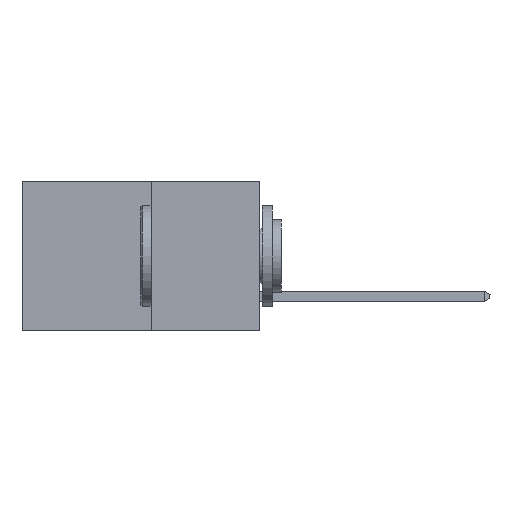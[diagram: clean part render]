
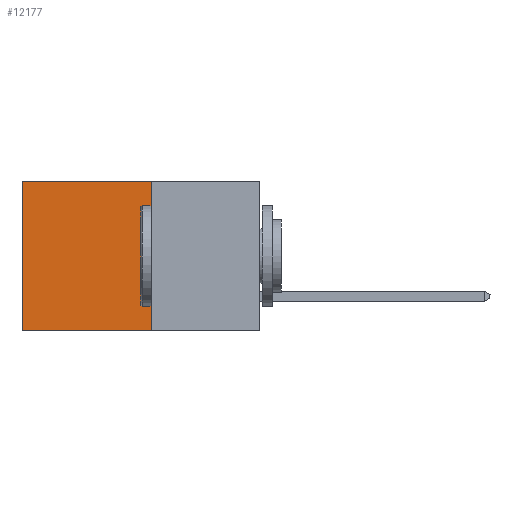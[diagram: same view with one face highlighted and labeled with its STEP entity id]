
A CAD part, left-side view. The second image highlights one B-rep face of the part: STEP entity #12177.
In plain terms, the highlighted planar face has unit normal (-1, 0, 0).
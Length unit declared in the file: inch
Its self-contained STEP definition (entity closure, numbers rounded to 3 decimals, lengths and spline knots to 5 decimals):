
#56 = LINE ( 'NONE', #4980, #15350 ) ;
#173 = VERTEX_POINT ( 'NONE', #7749 ) ;
#834 = ORIENTED_EDGE ( 'NONE', *, *, #2301, .F. ) ;
#1101 = PLANE ( 'NONE',  #8756 ) ;
#1112 = DIRECTION ( 'NONE',  ( 0., 0., -1. ) ) ;
#1713 = LINE ( 'NONE', #13297, #14385 ) ;
#1985 = EDGE_LOOP ( 'NONE', ( #5039, #834, #10351, #9979 ) ) ;
#2301 = EDGE_CURVE ( 'NONE', #8373, #12893, #13378, .T. ) ;
#2824 = FACE_OUTER_BOUND ( 'NONE', #1985, .T. ) ;
#4960 = DIRECTION ( 'NONE',  ( 1., 0., 0. ) ) ;
#4980 = CARTESIAN_POINT ( 'NONE',  ( 0.277, 0.27, 0. ) ) ;
#5039 = ORIENTED_EDGE ( 'NONE', *, *, #15071, .T. ) ;
#6705 = DIRECTION ( 'NONE',  ( 0., 1., 0. ) ) ;
#7002 = LINE ( 'NONE', #14675, #13492 ) ;
#7749 = CARTESIAN_POINT ( 'NONE',  ( 0.277, 0.59, 0. ) ) ;
#8121 = VERTEX_POINT ( 'NONE', #11681 ) ;
#8373 = VERTEX_POINT ( 'NONE', #9396 ) ;
#8756 = AXIS2_PLACEMENT_3D ( 'NONE', #12254, #4960, #13470 ) ;
#9396 = CARTESIAN_POINT ( 'NONE',  ( 0.277, 0.27, -0.37 ) ) ;
#9979 = ORIENTED_EDGE ( 'NONE', *, *, #11535, .T. ) ;
#10121 = VECTOR ( 'NONE', #6705, 39.37008 ) ;
#10351 = ORIENTED_EDGE ( 'NONE', *, *, #14503, .F. ) ;
#11165 = CARTESIAN_POINT ( 'NONE',  ( 0.277, 0.59, -0.37 ) ) ;
#11535 = EDGE_CURVE ( 'NONE', #8121, #173, #56, .T. ) ;
#11681 = CARTESIAN_POINT ( 'NONE',  ( 0.277, 0.27, 0. ) ) ;
#12177 = ADVANCED_FACE ( 'NONE', ( #2824 ), #1101, .F. ) ;
#12254 = CARTESIAN_POINT ( 'NONE',  ( 0.277, 0.27, -0.37 ) ) ;
#12893 = VERTEX_POINT ( 'NONE', #11165 ) ;
#13297 = CARTESIAN_POINT ( 'NONE',  ( 0.277, 0.59, -0.37 ) ) ;
#13378 = LINE ( 'NONE', #13827, #10121 ) ;
#13470 = DIRECTION ( 'NONE',  ( 0., 0., -1. ) ) ;
#13492 = VECTOR ( 'NONE', #1112, 39.37008 ) ;
#13827 = CARTESIAN_POINT ( 'NONE',  ( 0.277, 0.27, -0.37 ) ) ;
#14385 = VECTOR ( 'NONE', #14504, 39.37008 ) ;
#14503 = EDGE_CURVE ( 'NONE', #8121, #8373, #7002, .T. ) ;
#14504 = DIRECTION ( 'NONE',  ( 0., 0., -1. ) ) ;
#14675 = CARTESIAN_POINT ( 'NONE',  ( 0.277, 0.27, -0.37 ) ) ;
#14681 = DIRECTION ( 'NONE',  ( 0., 1., 0. ) ) ;
#15071 = EDGE_CURVE ( 'NONE', #173, #12893, #1713, .T. ) ;
#15350 = VECTOR ( 'NONE', #14681, 39.37008 ) ;
